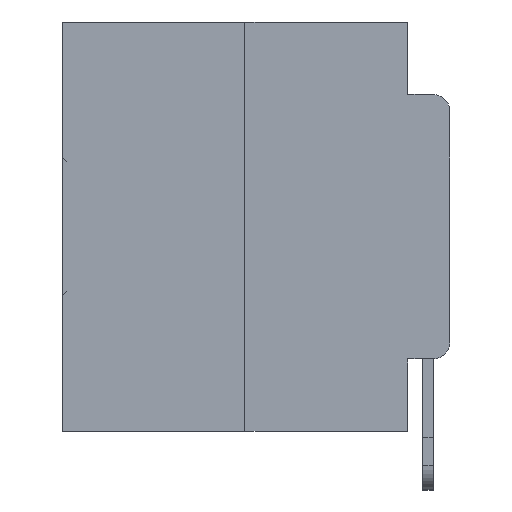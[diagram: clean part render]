
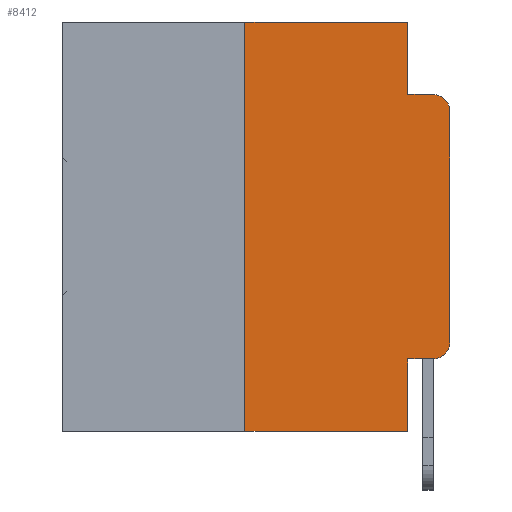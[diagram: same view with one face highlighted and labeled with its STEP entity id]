
A CAD part, left-side view. The second image highlights one B-rep face of the part: STEP entity #8412.
In plain terms, the highlighted planar face has unit normal (-1, 0, 0).
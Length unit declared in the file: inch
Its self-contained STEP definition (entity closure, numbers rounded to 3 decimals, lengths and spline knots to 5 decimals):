
#920 = LINE ( 'NONE', #21906, #20432 ) ;
#1079 = VECTOR ( 'NONE', #3380, 39.37008 ) ;
#1157 = CARTESIAN_POINT ( 'NONE',  ( 0., 0.473, 0. ) ) ;
#1594 = FACE_OUTER_BOUND ( 'NONE', #23017, .T. ) ;
#1673 = CARTESIAN_POINT ( 'NONE',  ( 0., 0.02, -0.4115 ) ) ;
#1984 = VERTEX_POINT ( 'NONE', #1673 ) ;
#2458 = LINE ( 'NONE', #13936, #8636 ) ;
#2645 = LINE ( 'NONE', #15631, #28418 ) ;
#2767 = VERTEX_POINT ( 'NONE', #15872 ) ;
#2991 = EDGE_CURVE ( 'NONE', #2767, #9700, #2645, .T. ) ;
#3019 = DIRECTION ( 'NONE',  ( -1., 0., 0. ) ) ;
#3380 = DIRECTION ( 'NONE',  ( 0., 0., -1. ) ) ;
#3498 = DIRECTION ( 'NONE',  ( 0., 0., 1. ) ) ;
#3806 = DIRECTION ( 'NONE',  ( 1., 0., 0. ) ) ;
#5107 = CARTESIAN_POINT ( 'NONE',  ( 0., 0.25, 0. ) ) ;
#5270 = VECTOR ( 'NONE', #30893, 39.37008 ) ;
#5408 = LINE ( 'NONE', #21832, #23749 ) ;
#6127 = CARTESIAN_POINT ( 'NONE',  ( 0., 0.02, -0.3915 ) ) ;
#7323 = AXIS2_PLACEMENT_3D ( 'NONE', #6127, #23541, #8736 ) ;
#7939 = EDGE_CURVE ( 'NONE', #19968, #27704, #2458, .T. ) ;
#8412 = ADVANCED_FACE ( 'NONE', ( #1594 ), #31028, .F. ) ;
#8499 = CARTESIAN_POINT ( 'NONE',  ( 0., 0.051, -0.4115 ) ) ;
#8636 = VECTOR ( 'NONE', #3498, 39.37008 ) ;
#8736 = DIRECTION ( 'NONE',  ( 0., 0., -1. ) ) ;
#8913 = CARTESIAN_POINT ( 'NONE',  ( 0., 0.051, -0.4115 ) ) ;
#9424 = ORIENTED_EDGE ( 'NONE', *, *, #21250, .F. ) ;
#9673 = EDGE_CURVE ( 'NONE', #27704, #17933, #11011, .T. ) ;
#9700 = VERTEX_POINT ( 'NONE', #10959 ) ;
#9741 = ORIENTED_EDGE ( 'NONE', *, *, #2991, .T. ) ;
#9749 = CIRCLE ( 'NONE', #7323, 0.02 ) ;
#10107 = ORIENTED_EDGE ( 'NONE', *, *, #27722, .F. ) ;
#10596 = ORIENTED_EDGE ( 'NONE', *, *, #19642, .F. ) ;
#10639 = ORIENTED_EDGE ( 'NONE', *, *, #18063, .F. ) ;
#10728 = ORIENTED_EDGE ( 'NONE', *, *, #15133, .F. ) ;
#10736 = CARTESIAN_POINT ( 'NONE',  ( 0., 0., -0.3915 ) ) ;
#10939 = VERTEX_POINT ( 'NONE', #5107 ) ;
#10959 = CARTESIAN_POINT ( 'NONE',  ( 0., 0.051, -0.5 ) ) ;
#11011 = CIRCLE ( 'NONE', #28672, 0.02 ) ;
#11418 = ORIENTED_EDGE ( 'NONE', *, *, #9673, .T. ) ;
#11484 = ORIENTED_EDGE ( 'NONE', *, *, #7939, .T. ) ;
#12442 = CARTESIAN_POINT ( 'NONE',  ( 0., 0., -0.1085 ) ) ;
#12783 = DIRECTION ( 'NONE',  ( 0., -1., 0. ) ) ;
#13184 = CARTESIAN_POINT ( 'NONE',  ( 0., 0.051, 0. ) ) ;
#13936 = CARTESIAN_POINT ( 'NONE',  ( 0., 0., 0. ) ) ;
#15133 = EDGE_CURVE ( 'NONE', #10939, #29097, #24390, .T. ) ;
#15631 = CARTESIAN_POINT ( 'NONE',  ( 0., 0.473, -0.5 ) ) ;
#15872 = CARTESIAN_POINT ( 'NONE',  ( 0., 0.25, -0.5 ) ) ;
#16209 = CARTESIAN_POINT ( 'NONE',  ( 0., 0.051, 0. ) ) ;
#16429 = DIRECTION ( 'NONE',  ( 0., -1., 0. ) ) ;
#16702 = LINE ( 'NONE', #19907, #22370 ) ;
#17091 = DIRECTION ( 'NONE',  ( 0., 0., -1. ) ) ;
#17933 = VERTEX_POINT ( 'NONE', #25405 ) ;
#18063 = EDGE_CURVE ( 'NONE', #29097, #28992, #21326, .T. ) ;
#18335 = CARTESIAN_POINT ( 'NONE',  ( 0., 0.02, -0.1085 ) ) ;
#19255 = LINE ( 'NONE', #8913, #24907 ) ;
#19486 = DIRECTION ( 'NONE',  ( 0., -1., 0. ) ) ;
#19642 = EDGE_CURVE ( 'NONE', #28992, #17933, #920, .T. ) ;
#19907 = CARTESIAN_POINT ( 'NONE',  ( 0., 0.25, 0. ) ) ;
#19968 = VERTEX_POINT ( 'NONE', #10736 ) ;
#20432 = VECTOR ( 'NONE', #19486, 39.37008 ) ;
#20717 = DIRECTION ( 'NONE',  ( 0., 0., -1. ) ) ;
#20941 = VERTEX_POINT ( 'NONE', #8499 ) ;
#21250 = EDGE_CURVE ( 'NONE', #20941, #9700, #5408, .T. ) ;
#21326 = LINE ( 'NONE', #16209, #1079 ) ;
#21452 = DIRECTION ( 'NONE',  ( 0., 0., -1. ) ) ;
#21832 = CARTESIAN_POINT ( 'NONE',  ( 0., 0.051, 0. ) ) ;
#21906 = CARTESIAN_POINT ( 'NONE',  ( 0., 0.051, -0.0885 ) ) ;
#22347 = DIRECTION ( 'NONE',  ( 0., 0., 1. ) ) ;
#22370 = VECTOR ( 'NONE', #22347, 39.37008 ) ;
#22563 = CARTESIAN_POINT ( 'NONE',  ( 0., 0.051, -0.0885 ) ) ;
#23017 = EDGE_LOOP ( 'NONE', ( #11484, #11418, #10596, #10639, #10728, #10107, #9741, #9424, #24040, #24366 ) ) ;
#23541 = DIRECTION ( 'NONE',  ( -1., 0., 0. ) ) ;
#23749 = VECTOR ( 'NONE', #17091, 39.37008 ) ;
#24040 = ORIENTED_EDGE ( 'NONE', *, *, #29360, .T. ) ;
#24320 = EDGE_CURVE ( 'NONE', #1984, #19968, #9749, .T. ) ;
#24366 = ORIENTED_EDGE ( 'NONE', *, *, #24320, .T. ) ;
#24390 = LINE ( 'NONE', #28499, #5270 ) ;
#24907 = VECTOR ( 'NONE', #16429, 39.37008 ) ;
#25405 = CARTESIAN_POINT ( 'NONE',  ( 0., 0.02, -0.0885 ) ) ;
#27704 = VERTEX_POINT ( 'NONE', #12442 ) ;
#27722 = EDGE_CURVE ( 'NONE', #2767, #10939, #16702, .T. ) ;
#28418 = VECTOR ( 'NONE', #12783, 39.37008 ) ;
#28499 = CARTESIAN_POINT ( 'NONE',  ( 0., 0.473, 0. ) ) ;
#28672 = AXIS2_PLACEMENT_3D ( 'NONE', #18335, #3019, #20717 ) ;
#28992 = VERTEX_POINT ( 'NONE', #22563 ) ;
#29097 = VERTEX_POINT ( 'NONE', #13184 ) ;
#29360 = EDGE_CURVE ( 'NONE', #20941, #1984, #19255, .T. ) ;
#29654 = AXIS2_PLACEMENT_3D ( 'NONE', #1157, #3806, #21452 ) ;
#30893 = DIRECTION ( 'NONE',  ( 0., -1., 0. ) ) ;
#31028 = PLANE ( 'NONE',  #29654 ) ;
